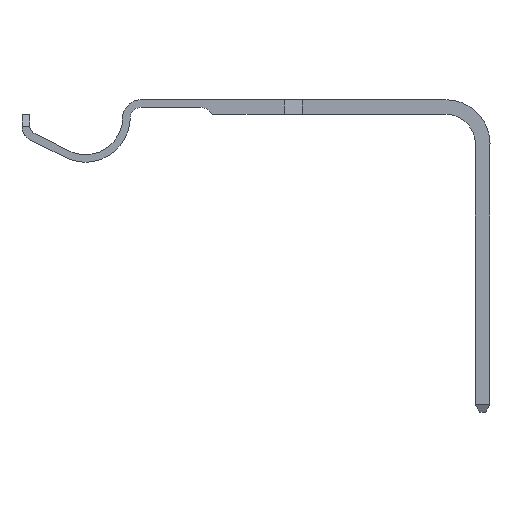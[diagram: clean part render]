
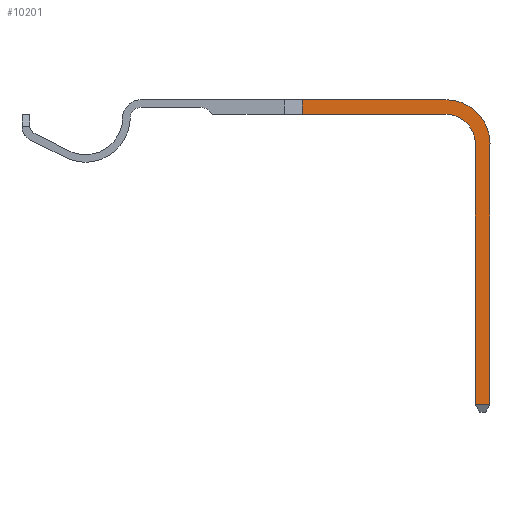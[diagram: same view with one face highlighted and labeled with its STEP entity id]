
A CAD part, left-side view. The second image highlights one B-rep face of the part: STEP entity #10201.
In plain terms, the highlighted face is planar.
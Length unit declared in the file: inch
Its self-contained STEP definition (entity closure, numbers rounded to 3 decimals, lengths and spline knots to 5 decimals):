
#1300 = VERTEX_POINT ( 'NONE', #14944 ) ;
#1393 = FACE_OUTER_BOUND ( 'NONE', #1893, .T. ) ;
#1480 = VECTOR ( 'NONE', #8670, 39.37008 ) ;
#1893 = EDGE_LOOP ( 'NONE', ( #15147, #8785, #23650, #20913, #15428, #13777, #20308, #19946 ) ) ;
#2258 = LINE ( 'NONE', #25131, #27145 ) ;
#2342 = EDGE_CURVE ( 'NONE', #29292, #1300, #7474, .T. ) ;
#3193 = AXIS2_PLACEMENT_3D ( 'NONE', #4411, #21345, #6919 ) ;
#3247 = EDGE_CURVE ( 'NONE', #21611, #15067, #24301, .T. ) ;
#3929 = DIRECTION ( 'NONE',  ( 0., 0., -1. ) ) ;
#4411 = CARTESIAN_POINT ( 'NONE',  ( 0.85571, 0.0875, -0.0125 ) ) ;
#4529 = CARTESIAN_POINT ( 'NONE',  ( 0.85571, 0.0125, -0.0125 ) ) ;
#5010 = CIRCLE ( 'NONE', #18566, 0.075 ) ;
#5166 = CARTESIAN_POINT ( 'NONE',  ( 0.85571, 0.0875, -0.0125 ) ) ;
#5255 = VERTEX_POINT ( 'NONE', #16928 ) ;
#6042 = DIRECTION ( 'NONE',  ( -1., 0., 0. ) ) ;
#6364 = CARTESIAN_POINT ( 'NONE',  ( 0.85571, 0.0375, -0.0125 ) ) ;
#6542 = VERTEX_POINT ( 'NONE', #4529 ) ;
#6842 = AXIS2_PLACEMENT_3D ( 'NONE', #5166, #22065, #7676 ) ;
#6919 = DIRECTION ( 'NONE',  ( 1., 0., 0. ) ) ;
#7474 = LINE ( 'NONE', #26494, #25818 ) ;
#7676 = DIRECTION ( 'NONE',  ( 1., 0., 0. ) ) ;
#8405 = DIRECTION ( 'NONE',  ( 0., -1., 0. ) ) ;
#8670 = DIRECTION ( 'NONE',  ( 1., 0., 0. ) ) ;
#8785 = ORIENTED_EDGE ( 'NONE', *, *, #22601, .T. ) ;
#9110 = CARTESIAN_POINT ( 'NONE',  ( 0.61115, 0.0125, -0.0125 ) ) ;
#10085 = VECTOR ( 'NONE', #25930, 39.37008 ) ;
#10201 = ADVANCED_FACE ( 'NONE', ( #1393 ), #16540, .F. ) ;
#10854 = CIRCLE ( 'NONE', #6842, 0.05 ) ;
#10994 = CARTESIAN_POINT ( 'NONE',  ( 0.85571, 0.532, -0.0125 ) ) ;
#11487 = VERTEX_POINT ( 'NONE', #9110 ) ;
#11840 = EDGE_CURVE ( 'NONE', #6542, #11487, #29171, .T. ) ;
#13315 = CARTESIAN_POINT ( 'NONE',  ( 0.58021, 0.0125, -0.0125 ) ) ;
#13530 = CARTESIAN_POINT ( 'NONE',  ( 0.58021, 0.0375, -0.0125 ) ) ;
#13777 = ORIENTED_EDGE ( 'NONE', *, *, #21059, .T. ) ;
#14756 = EDGE_CURVE ( 'NONE', #15067, #29292, #10854, .T. ) ;
#14944 = CARTESIAN_POINT ( 'NONE',  ( 0.90571, 0.532, -0.0125 ) ) ;
#15067 = VERTEX_POINT ( 'NONE', #6364 ) ;
#15147 = ORIENTED_EDGE ( 'NONE', *, *, #2342, .T. ) ;
#15428 = ORIENTED_EDGE ( 'NONE', *, *, #11840, .T. ) ;
#15569 = EDGE_CURVE ( 'NONE', #5255, #6542, #5010, .T. ) ;
#16267 = EDGE_CURVE ( 'NONE', #26627, #5255, #2258, .T. ) ;
#16540 = PLANE ( 'NONE',  #3193 ) ;
#16928 = CARTESIAN_POINT ( 'NONE',  ( 0.93071, 0.0875, -0.0125 ) ) ;
#17238 = DIRECTION ( 'NONE',  ( 1., 0., 0. ) ) ;
#17959 = VECTOR ( 'NONE', #17238, 39.37008 ) ;
#18487 = CARTESIAN_POINT ( 'NONE',  ( 0.85571, 0.0875, -0.0125 ) ) ;
#18566 = AXIS2_PLACEMENT_3D ( 'NONE', #18487, #3929, #20891 ) ;
#19946 = ORIENTED_EDGE ( 'NONE', *, *, #14756, .T. ) ;
#20308 = ORIENTED_EDGE ( 'NONE', *, *, #3247, .T. ) ;
#20660 = DIRECTION ( 'NONE',  ( 0., 1., 0. ) ) ;
#20891 = DIRECTION ( 'NONE',  ( 1., 0., 0. ) ) ;
#20913 = ORIENTED_EDGE ( 'NONE', *, *, #15569, .T. ) ;
#21059 = EDGE_CURVE ( 'NONE', #11487, #21611, #22834, .T. ) ;
#21345 = DIRECTION ( 'NONE',  ( 0., 0., 1. ) ) ;
#21611 = VERTEX_POINT ( 'NONE', #21824 ) ;
#21824 = CARTESIAN_POINT ( 'NONE',  ( 0.61115, 0.0375, -0.0125 ) ) ;
#22065 = DIRECTION ( 'NONE',  ( 0., 0., 1. ) ) ;
#22601 = EDGE_CURVE ( 'NONE', #1300, #26627, #27130, .T. ) ;
#22834 = LINE ( 'NONE', #23786, #10085 ) ;
#22906 = VECTOR ( 'NONE', #6042, 39.37008 ) ;
#23650 = ORIENTED_EDGE ( 'NONE', *, *, #16267, .T. ) ;
#23786 = CARTESIAN_POINT ( 'NONE',  ( 0.61115, 0.0875, -0.0125 ) ) ;
#24301 = LINE ( 'NONE', #13530, #17959 ) ;
#24799 = CARTESIAN_POINT ( 'NONE',  ( 0.90571, 0.0875, -0.0125 ) ) ;
#25131 = CARTESIAN_POINT ( 'NONE',  ( 0.93071, 0.0875, -0.0125 ) ) ;
#25818 = VECTOR ( 'NONE', #20660, 39.37008 ) ;
#25930 = DIRECTION ( 'NONE',  ( 0., 1., 0. ) ) ;
#26494 = CARTESIAN_POINT ( 'NONE',  ( 0.90571, 0.0875, -0.0125 ) ) ;
#26627 = VERTEX_POINT ( 'NONE', #28428 ) ;
#27130 = LINE ( 'NONE', #10994, #1480 ) ;
#27145 = VECTOR ( 'NONE', #8405, 39.37008 ) ;
#28428 = CARTESIAN_POINT ( 'NONE',  ( 0.93071, 0.532, -0.0125 ) ) ;
#29171 = LINE ( 'NONE', #13315, #22906 ) ;
#29292 = VERTEX_POINT ( 'NONE', #24799 ) ;
